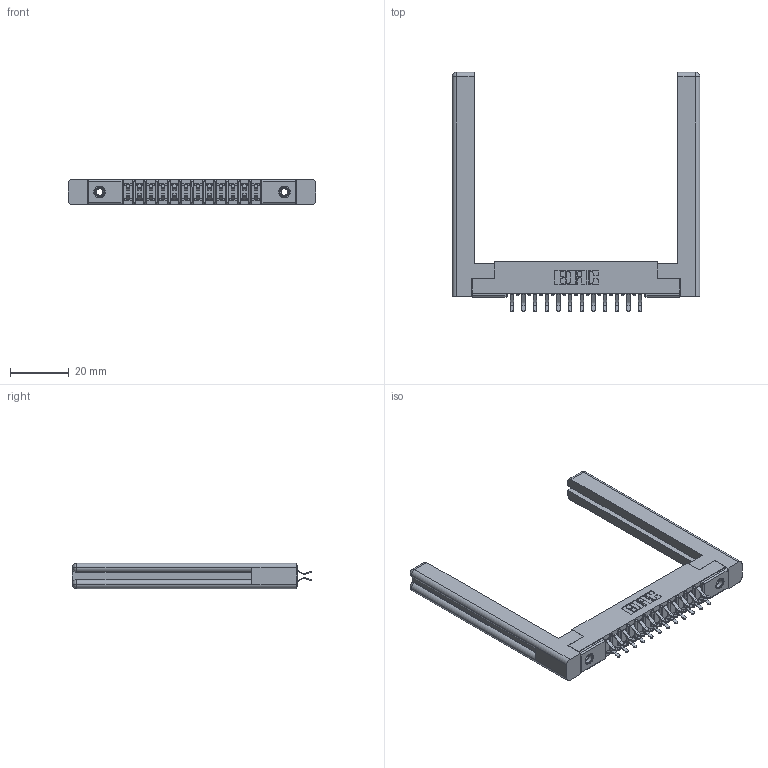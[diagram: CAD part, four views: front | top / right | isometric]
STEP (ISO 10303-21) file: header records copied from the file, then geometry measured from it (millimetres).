
FILE_DESCRIPTION (( 'STEP AP203' ), '1' );
FILE_NAME ('307-024-456-258.STEP', '2020-09-29T05:25:36', ( '' ), ( '' ), 'SwSTEP 2.0', 'SolidWorks 2020', '' );
FILE_SCHEMA (( 'CONFIG_CONTROL_DESIGN' ));
Length unit declared in the file: inch
Products named in the file (5): 345-250-001_345-250-001-102; 307-290-001_556; 307-220-058; 307 Part_.156 Dia Mounting Holes; 307-024-456-258
Assembly tree (29 placements, depth 2):
  307-024-456-258
    307 Part_.156 Dia Mounting Holes
    307-290-001_556  x24
    307-220-058  x2
    345-250-001_345-250-001-102  x2
Bounding box: 84.18 x 81.28 x 8.71 mm (x, y, z)
Volume: 13189.4 mm3; surface area: 14263.2 mm2
Topology: 29 solids, 29 shells, 1473 faces, 4085 edges, 2642 vertices
Faces by surface type: plane 946, cylinder 477, sphere 26, torus 12, cone 12
Entity records: 17107 total; most frequent: CARTESIAN_POINT 2827, DIRECTION 2740, ORIENTED_EDGE 2740, EDGE_CURVE 1370, LINE 1034, VECTOR 1034, VERTEX_POINT 886, AXIS2_PLACEMENT_3D 853
